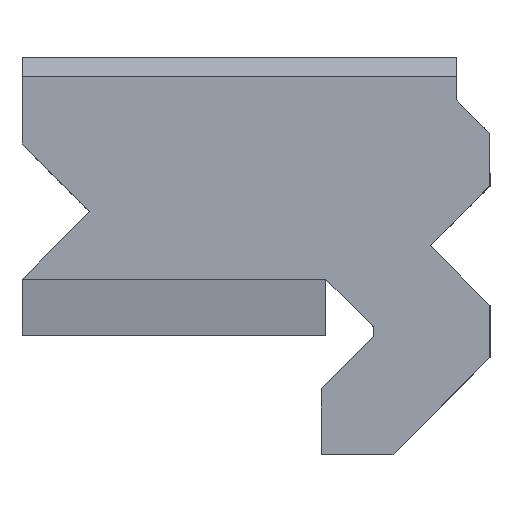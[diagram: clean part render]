
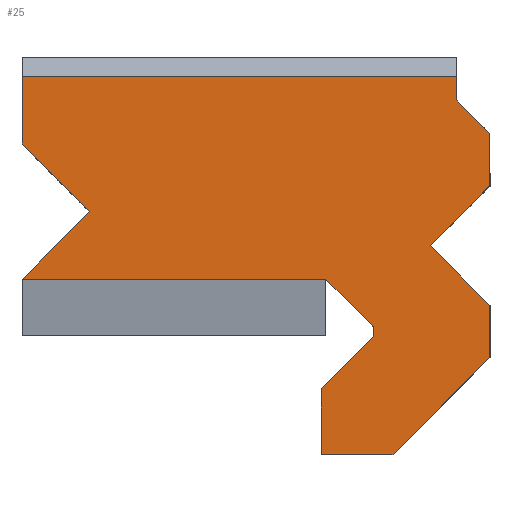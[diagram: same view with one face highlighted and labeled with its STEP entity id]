
A CAD part, top view. The second image highlights one B-rep face of the part: STEP entity #25.
In plain terms, the highlighted planar face has unit normal (0, 0, 1).
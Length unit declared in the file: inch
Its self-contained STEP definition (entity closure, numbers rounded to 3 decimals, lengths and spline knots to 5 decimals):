
#8 = VERTEX_POINT ( 'NONE', #177 ) ;
#16 = VECTOR ( 'NONE', #437, 39.37008 ) ;
#20 = CARTESIAN_POINT ( 'NONE',  ( 0.66475, 0.18014, 0.02825 ) ) ;
#22 = EDGE_CURVE ( 'NONE', #606, #724, #350, .T. ) ;
#25 = ADVANCED_FACE ( 'NONE', ( #210 ), #997, .F. ) ;
#56 = CARTESIAN_POINT ( 'NONE',  ( 0.78975, 0.30514, 0.02825 ) ) ;
#57 = VERTEX_POINT ( 'NONE', #391 ) ;
#64 = LINE ( 'NONE', #195, #903 ) ;
#65 = CARTESIAN_POINT ( 'NONE',  ( 0.54575, 0.0105, 0.02825 ) ) ;
#70 = ORIENTED_EDGE ( 'NONE', *, *, #182, .F. ) ;
#73 = LINE ( 'NONE', #950, #1049 ) ;
#78 = VERTEX_POINT ( 'NONE', #478 ) ;
#93 = DIRECTION ( 'NONE',  ( -0.707, -0.707, 0. ) ) ;
#94 = LINE ( 'NONE', #1025, #829 ) ;
#106 = ORIENTED_EDGE ( 'NONE', *, *, #890, .T. ) ;
#113 = CARTESIAN_POINT ( 'NONE',  ( 0.71904, 0.53464, 0.02825 ) ) ;
#115 = CARTESIAN_POINT ( 'NONE',  ( 0.78975, -0.054, 0.02825 ) ) ;
#119 = ORIENTED_EDGE ( 'NONE', *, *, #995, .T. ) ;
#132 = VERTEX_POINT ( 'NONE', #304 ) ;
#144 = CARTESIAN_POINT ( 'NONE',  ( 0.78975, 0.30514, 0.02825 ) ) ;
#159 = ORIENTED_EDGE ( 'NONE', *, *, #536, .F. ) ;
#162 = ORIENTED_EDGE ( 'NONE', *, *, #1053, .T. ) ;
#164 = VECTOR ( 'NONE', #416, 39.37008 ) ;
#171 = ORIENTED_EDGE ( 'NONE', *, *, #754, .F. ) ;
#177 = CARTESIAN_POINT ( 'NONE',  ( 0.43675, -0.257, 0.02825 ) ) ;
#179 = DIRECTION ( 'NONE',  ( 0.707, -0.707, 0. ) ) ;
#181 = CARTESIAN_POINT ( 'NONE',  ( 0.71904, 0.485, 0.02825 ) ) ;
#182 = EDGE_CURVE ( 'NONE', #724, #8, #1093, .T. ) ;
#195 = CARTESIAN_POINT ( 'NONE',  ( 2.32533, 0.53464, 0.02825 ) ) ;
#203 = VERTEX_POINT ( 'NONE', #144 ) ;
#210 = FACE_OUTER_BOUND ( 'NONE', #900, .T. ) ;
#213 = CARTESIAN_POINT ( 'NONE',  ( 0.71904, 0.485, 0.02825 ) ) ;
#246 = LINE ( 'NONE', #431, #285 ) ;
#258 = LINE ( 'NONE', #444, #283 ) ;
#272 = EDGE_CURVE ( 'NONE', #650, #415, #73, .T. ) ;
#275 = EDGE_CURVE ( 'NONE', #381, #78, #518, .T. ) ;
#283 = VECTOR ( 'NONE', #179, 39.37008 ) ;
#285 = VECTOR ( 'NONE', #681, 39.37008 ) ;
#293 = VERTEX_POINT ( 'NONE', #328 ) ;
#304 = CARTESIAN_POINT ( 'NONE',  ( 0.54575, 0.0105, 0.02825 ) ) ;
#308 = ORIENTED_EDGE ( 'NONE', *, *, #941, .F. ) ;
#311 = ORIENTED_EDGE ( 'NONE', *, *, #272, .T. ) ;
#328 = CARTESIAN_POINT ( 'NONE',  ( -0.18975, 0.39284, 0.02825 ) ) ;
#343 = EDGE_CURVE ( 'NONE', #942, #203, #577, .T. ) ;
#347 = LINE ( 'NONE', #20, #712 ) ;
#350 = LINE ( 'NONE', #560, #703 ) ;
#352 = CARTESIAN_POINT ( 'NONE',  ( 0.44625, 0.11, 0.02825 ) ) ;
#355 = CARTESIAN_POINT ( 'NONE',  ( 0.43675, -0.1195, 0.02825 ) ) ;
#363 = DIRECTION ( 'NONE',  ( 0., -1., 0. ) ) ;
#366 = LINE ( 'NONE', #65, #164 ) ;
#373 = DIRECTION ( 'NONE',  ( 0., -1., 0. ) ) ;
#380 = ORIENTED_EDGE ( 'NONE', *, *, #682, .F. ) ;
#381 = VERTEX_POINT ( 'NONE', #355 ) ;
#391 = CARTESIAN_POINT ( 'NONE',  ( -0.18975, 0.53464, 0.02825 ) ) ;
#403 = CARTESIAN_POINT ( 'NONE',  ( -0.04833, 0.25142, 0.02825 ) ) ;
#415 = VERTEX_POINT ( 'NONE', #705 ) ;
#416 = DIRECTION ( 'NONE',  ( 0., 1., 0. ) ) ;
#422 = ORIENTED_EDGE ( 'NONE', *, *, #1120, .F. ) ;
#431 = CARTESIAN_POINT ( 'NONE',  ( -0.18975, 0.11, 0.02825 ) ) ;
#437 = DIRECTION ( 'NONE',  ( 0.707, -0.707, 0. ) ) ;
#444 = CARTESIAN_POINT ( 'NONE',  ( -0.04833, 0.25142, 0.02825 ) ) ;
#455 = DIRECTION ( 'NONE',  ( -0.707, 0.707, 0. ) ) ;
#457 = DIRECTION ( 'NONE',  ( -1., 0., 0. ) ) ;
#461 = CARTESIAN_POINT ( 'NONE',  ( 0.78975, 0.05514, 0.02825 ) ) ;
#462 = VECTOR ( 'NONE', #706, 39.37008 ) ;
#471 = DIRECTION ( 'NONE',  ( 0., 0., -1. ) ) ;
#476 = ORIENTED_EDGE ( 'NONE', *, *, #22, .F. ) ;
#478 = CARTESIAN_POINT ( 'NONE',  ( 0.54575, -0.0105, 0.02825 ) ) ;
#481 = LINE ( 'NONE', #56, #713 ) ;
#494 = EDGE_CURVE ( 'NONE', #978, #57, #64, .T. ) ;
#518 = LINE ( 'NONE', #670, #934 ) ;
#525 = DIRECTION ( 'NONE',  ( 0., -1., 0. ) ) ;
#536 = EDGE_CURVE ( 'NONE', #978, #539, #1102, .T. ) ;
#537 = CARTESIAN_POINT ( 'NONE',  ( 2.32533, 0.57464, 0.02825 ) ) ;
#539 = VERTEX_POINT ( 'NONE', #213 ) ;
#560 = CARTESIAN_POINT ( 'NONE',  ( 0.58675, -0.257, 0.02825 ) ) ;
#570 = VERTEX_POINT ( 'NONE', #1075 ) ;
#577 = LINE ( 'NONE', #772, #752 ) ;
#595 = LINE ( 'NONE', #115, #462 ) ;
#599 = CARTESIAN_POINT ( 'NONE',  ( 0.78975, 0.41429, 0.02825 ) ) ;
#606 = VERTEX_POINT ( 'NONE', #1001 ) ;
#623 = DIRECTION ( 'NONE',  ( -0.707, 0.707, 0. ) ) ;
#630 = EDGE_CURVE ( 'NONE', #570, #203, #481, .T. ) ;
#650 = VERTEX_POINT ( 'NONE', #403 ) ;
#664 = VECTOR ( 'NONE', #455, 39.37008 ) ;
#669 = ORIENTED_EDGE ( 'NONE', *, *, #494, .T. ) ;
#670 = CARTESIAN_POINT ( 'NONE',  ( 0.43675, -0.1195, 0.02825 ) ) ;
#671 = DIRECTION ( 'NONE',  ( -0.707, -0.707, 0. ) ) ;
#681 = DIRECTION ( 'NONE',  ( -1., 0., 0. ) ) ;
#682 = EDGE_CURVE ( 'NONE', #78, #132, #366, .T. ) ;
#691 = VECTOR ( 'NONE', #920, 39.37008 ) ;
#699 = LINE ( 'NONE', #979, #915 ) ;
#703 = VECTOR ( 'NONE', #93, 39.37008 ) ;
#705 = CARTESIAN_POINT ( 'NONE',  ( -0.18975, 0.11, 0.02825 ) ) ;
#706 = DIRECTION ( 'NONE',  ( 0., -1., 0. ) ) ;
#710 = ORIENTED_EDGE ( 'NONE', *, *, #630, .T. ) ;
#711 = CARTESIAN_POINT ( 'NONE',  ( 0.44625, 0.11, 0.02825 ) ) ;
#712 = VECTOR ( 'NONE', #623, 39.37008 ) ;
#713 = VECTOR ( 'NONE', #746, 39.37008 ) ;
#724 = VERTEX_POINT ( 'NONE', #744 ) ;
#744 = CARTESIAN_POINT ( 'NONE',  ( 0.58675, -0.257, 0.02825 ) ) ;
#746 = DIRECTION ( 'NONE',  ( 0.707, 0.707, 0. ) ) ;
#750 = ORIENTED_EDGE ( 'NONE', *, *, #343, .F. ) ;
#752 = VECTOR ( 'NONE', #525, 39.37008 ) ;
#753 = ORIENTED_EDGE ( 'NONE', *, *, #1014, .F. ) ;
#754 = EDGE_CURVE ( 'NONE', #928, #415, #246, .T. ) ;
#757 = DIRECTION ( 'NONE',  ( 0., 1., 0. ) ) ;
#772 = CARTESIAN_POINT ( 'NONE',  ( 0.78975, -0.054, 0.02825 ) ) ;
#791 = LINE ( 'NONE', #711, #664 ) ;
#823 = EDGE_CURVE ( 'NONE', #8, #381, #94, .T. ) ;
#829 = VECTOR ( 'NONE', #757, 39.37008 ) ;
#839 = ORIENTED_EDGE ( 'NONE', *, *, #275, .F. ) ;
#867 = ORIENTED_EDGE ( 'NONE', *, *, #823, .F. ) ;
#875 = VECTOR ( 'NONE', #373, 39.37008 ) ;
#890 = EDGE_CURVE ( 'NONE', #293, #650, #258, .T. ) ;
#895 = CARTESIAN_POINT ( 'NONE',  ( 0.71904, 0.485, 0.02825 ) ) ;
#900 = EDGE_LOOP ( 'NONE', ( #159, #669, #162, #106, #311, #171, #422, #380, #839, #867, #70, #476, #753, #119, #710, #750, #308 ) ) ;
#902 = AXIS2_PLACEMENT_3D ( 'NONE', #537, #471, #1059 ) ;
#903 = VECTOR ( 'NONE', #457, 39.37008 ) ;
#915 = VECTOR ( 'NONE', #363, 39.37008 ) ;
#920 = DIRECTION ( 'NONE',  ( -1., 0., 0. ) ) ;
#928 = VERTEX_POINT ( 'NONE', #352 ) ;
#934 = VECTOR ( 'NONE', #1020, 39.37008 ) ;
#941 = EDGE_CURVE ( 'NONE', #539, #942, #1007, .T. ) ;
#942 = VERTEX_POINT ( 'NONE', #599 ) ;
#950 = CARTESIAN_POINT ( 'NONE',  ( -0.18975, 0.11, 0.02825 ) ) ;
#978 = VERTEX_POINT ( 'NONE', #113 ) ;
#979 = CARTESIAN_POINT ( 'NONE',  ( -0.18975, 0.39284, 0.02825 ) ) ;
#995 = EDGE_CURVE ( 'NONE', #1005, #570, #347, .T. ) ;
#997 = PLANE ( 'NONE',  #902 ) ;
#1001 = CARTESIAN_POINT ( 'NONE',  ( 0.78975, -0.054, 0.02825 ) ) ;
#1005 = VERTEX_POINT ( 'NONE', #461 ) ;
#1007 = LINE ( 'NONE', #181, #16 ) ;
#1011 = CARTESIAN_POINT ( 'NONE',  ( 0.43675, -0.257, 0.02825 ) ) ;
#1014 = EDGE_CURVE ( 'NONE', #1005, #606, #595, .T. ) ;
#1020 = DIRECTION ( 'NONE',  ( 0.707, 0.707, 0. ) ) ;
#1025 = CARTESIAN_POINT ( 'NONE',  ( 0.43675, -0.257, 0.02825 ) ) ;
#1049 = VECTOR ( 'NONE', #671, 39.37008 ) ;
#1053 = EDGE_CURVE ( 'NONE', #57, #293, #699, .T. ) ;
#1059 = DIRECTION ( 'NONE',  ( -1., 0., 0. ) ) ;
#1075 = CARTESIAN_POINT ( 'NONE',  ( 0.66475, 0.18014, 0.02825 ) ) ;
#1093 = LINE ( 'NONE', #1011, #691 ) ;
#1102 = LINE ( 'NONE', #895, #875 ) ;
#1120 = EDGE_CURVE ( 'NONE', #132, #928, #791, .T. ) ;
